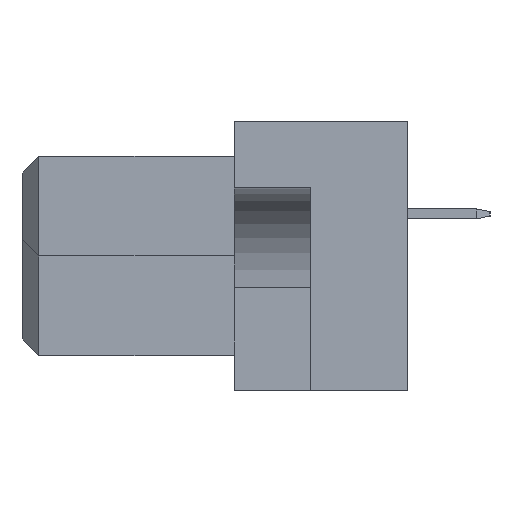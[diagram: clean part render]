
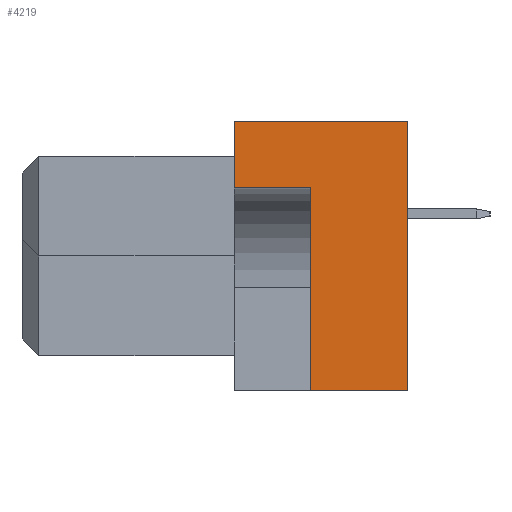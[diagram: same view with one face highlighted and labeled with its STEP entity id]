
A CAD part, left-side view. The second image highlights one B-rep face of the part: STEP entity #4219.
In plain terms, the highlighted planar face has unit normal (-1, 0, 0).
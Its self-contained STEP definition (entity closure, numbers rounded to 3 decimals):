
#1352 = EDGE_CURVE ( 'NONE', #2995, #8607, #15792, .T. ) ;
#2995 = VERTEX_POINT ( 'NONE', #16181 ) ;
#3302 = DIRECTION ( 'NONE',  ( 0., 0., 1. ) ) ;
#3407 = CARTESIAN_POINT ( 'NONE',  ( -47.5, 5.2, 4.05 ) ) ;
#3660 = FACE_OUTER_BOUND ( 'NONE', #17782, .T. ) ;
#4219 = ADVANCED_FACE ( 'NONE', ( #3660 ), #15918, .F. ) ;
#5970 = CARTESIAN_POINT ( 'NONE',  ( -47.5, 2.9, 2.05 ) ) ;
#6074 = VECTOR ( 'NONE', #3302, 1000. ) ;
#6095 = LINE ( 'NONE', #5970, #8181 ) ;
#6979 = VERTEX_POINT ( 'NONE', #23959 ) ;
#8181 = VECTOR ( 'NONE', #26607, 1000. ) ;
#8305 = VECTOR ( 'NONE', #19472, 1000. ) ;
#8607 = VERTEX_POINT ( 'NONE', #26355 ) ;
#9636 = CARTESIAN_POINT ( 'NONE',  ( -47.5, 0., 4.05 ) ) ;
#10672 = CARTESIAN_POINT ( 'NONE',  ( -47.5, 5.2, -4.05 ) ) ;
#10793 = DIRECTION ( 'NONE',  ( 0., -1., 0. ) ) ;
#11362 = CARTESIAN_POINT ( 'NONE',  ( -47.5, 2.9, 2.05 ) ) ;
#11468 = DIRECTION ( 'NONE',  ( 0., -1., 0. ) ) ;
#11931 = DIRECTION ( 'NONE',  ( 0., 0., 1. ) ) ;
#13568 = VERTEX_POINT ( 'NONE', #17778 ) ;
#13891 = CARTESIAN_POINT ( 'NONE',  ( -47.5, 5.2, 4.05 ) ) ;
#15041 = VERTEX_POINT ( 'NONE', #25812 ) ;
#15546 = LINE ( 'NONE', #21749, #6074 ) ;
#15792 = LINE ( 'NONE', #3407, #22292 ) ;
#15918 = PLANE ( 'NONE',  #22015 ) ;
#16181 = CARTESIAN_POINT ( 'NONE',  ( -47.5, 5.2, 4.05 ) ) ;
#16335 = ORIENTED_EDGE ( 'NONE', *, *, #1352, .F. ) ;
#16826 = VECTOR ( 'NONE', #10793, 1000. ) ;
#16841 = EDGE_CURVE ( 'NONE', #24258, #2995, #15546, .T. ) ;
#16924 = ORIENTED_EDGE ( 'NONE', *, *, #20949, .T. ) ;
#17017 = CARTESIAN_POINT ( 'NONE',  ( -47.5, 5.2, 2.05 ) ) ;
#17144 = LINE ( 'NONE', #10672, #16826 ) ;
#17778 = CARTESIAN_POINT ( 'NONE',  ( -47.5, 2.9, -4.05 ) ) ;
#17782 = EDGE_LOOP ( 'NONE', ( #19337, #19880, #21666, #22131, #16924, #16335 ) ) ;
#19337 = ORIENTED_EDGE ( 'NONE', *, *, #16841, .F. ) ;
#19472 = DIRECTION ( 'NONE',  ( 0., 1., 0. ) ) ;
#19734 = EDGE_CURVE ( 'NONE', #13568, #15041, #6095, .T. ) ;
#19805 = EDGE_CURVE ( 'NONE', #13568, #6979, #17144, .T. ) ;
#19880 = ORIENTED_EDGE ( 'NONE', *, *, #22677, .F. ) ;
#20949 = EDGE_CURVE ( 'NONE', #6979, #8607, #24339, .T. ) ;
#21358 = LINE ( 'NONE', #11362, #8305 ) ;
#21666 = ORIENTED_EDGE ( 'NONE', *, *, #19734, .F. ) ;
#21749 = CARTESIAN_POINT ( 'NONE',  ( -47.5, 5.2, 4.05 ) ) ;
#22015 = AXIS2_PLACEMENT_3D ( 'NONE', #13891, #22117, #25789 ) ;
#22117 = DIRECTION ( 'NONE',  ( 1., 0., 0. ) ) ;
#22131 = ORIENTED_EDGE ( 'NONE', *, *, #19805, .T. ) ;
#22292 = VECTOR ( 'NONE', #11468, 1000. ) ;
#22677 = EDGE_CURVE ( 'NONE', #15041, #24258, #21358, .T. ) ;
#23959 = CARTESIAN_POINT ( 'NONE',  ( -47.5, 0., -4.05 ) ) ;
#24258 = VERTEX_POINT ( 'NONE', #17017 ) ;
#24339 = LINE ( 'NONE', #9636, #25493 ) ;
#25493 = VECTOR ( 'NONE', #11931, 1000. ) ;
#25789 = DIRECTION ( 'NONE',  ( 0., 0., -1. ) ) ;
#25812 = CARTESIAN_POINT ( 'NONE',  ( -47.5, 2.9, 2.05 ) ) ;
#26355 = CARTESIAN_POINT ( 'NONE',  ( -47.5, 0., 4.05 ) ) ;
#26607 = DIRECTION ( 'NONE',  ( 0., 0., 1. ) ) ;
